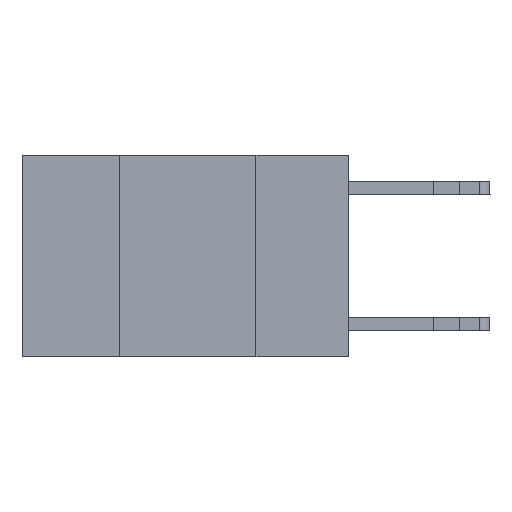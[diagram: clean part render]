
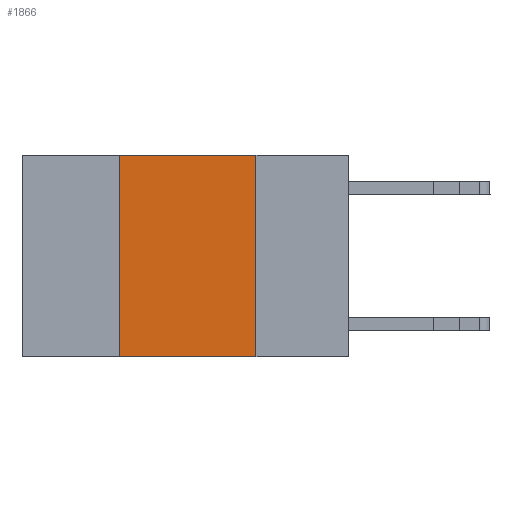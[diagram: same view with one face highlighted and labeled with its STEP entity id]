
A CAD part, left-side view. The second image highlights one B-rep face of the part: STEP entity #1866.
In plain terms, the highlighted planar face has unit normal (-1, 0, 0).
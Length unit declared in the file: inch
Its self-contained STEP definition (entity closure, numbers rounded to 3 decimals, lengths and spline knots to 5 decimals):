
#20 = CARTESIAN_POINT ( 'NONE',  ( 0., 0.42, 0. ) ) ;
#756 = ORIENTED_EDGE ( 'NONE', *, *, #8508, .F. ) ;
#1008 = LINE ( 'NONE', #17419, #14251 ) ;
#1150 = VERTEX_POINT ( 'NONE', #14821 ) ;
#1290 = LINE ( 'NONE', #5281, #10766 ) ;
#1866 = ADVANCED_FACE ( 'NONE', ( #12064 ), #17331, .F. ) ;
#2930 = EDGE_LOOP ( 'NONE', ( #5076, #9175, #756, #7237 ) ) ;
#4109 = CARTESIAN_POINT ( 'NONE',  ( 0., 0.17, 0. ) ) ;
#5074 = DIRECTION ( 'NONE',  ( 0., -1., 0. ) ) ;
#5076 = ORIENTED_EDGE ( 'NONE', *, *, #10309, .F. ) ;
#5144 = CARTESIAN_POINT ( 'NONE',  ( 0., 0.6, 0. ) ) ;
#5281 = CARTESIAN_POINT ( 'NONE',  ( 0., 0.6, -0.37 ) ) ;
#5461 = DIRECTION ( 'NONE',  ( 0., 0., -1. ) ) ;
#7237 = ORIENTED_EDGE ( 'NONE', *, *, #7477, .T. ) ;
#7477 = EDGE_CURVE ( 'NONE', #13614, #10065, #1290, .T. ) ;
#7656 = AXIS2_PLACEMENT_3D ( 'NONE', #5144, #17405, #13313 ) ;
#8288 = EDGE_CURVE ( 'NONE', #1150, #13953, #1008, .T. ) ;
#8508 = EDGE_CURVE ( 'NONE', #13614, #1150, #12174, .T. ) ;
#9175 = ORIENTED_EDGE ( 'NONE', *, *, #8288, .F. ) ;
#10065 = VERTEX_POINT ( 'NONE', #11707 ) ;
#10309 = EDGE_CURVE ( 'NONE', #13953, #10065, #12397, .T. ) ;
#10766 = VECTOR ( 'NONE', #12216, 39.37008 ) ;
#11707 = CARTESIAN_POINT ( 'NONE',  ( 0., 0.17, -0.37 ) ) ;
#12064 = FACE_OUTER_BOUND ( 'NONE', #2930, .T. ) ;
#12174 = LINE ( 'NONE', #20, #12218 ) ;
#12216 = DIRECTION ( 'NONE',  ( 0., -1., 0. ) ) ;
#12218 = VECTOR ( 'NONE', #16301, 39.37008 ) ;
#12397 = LINE ( 'NONE', #15380, #16010 ) ;
#13313 = DIRECTION ( 'NONE',  ( 0., 0., -1. ) ) ;
#13614 = VERTEX_POINT ( 'NONE', #16503 ) ;
#13953 = VERTEX_POINT ( 'NONE', #4109 ) ;
#14251 = VECTOR ( 'NONE', #5074, 39.37008 ) ;
#14821 = CARTESIAN_POINT ( 'NONE',  ( 0., 0.42, 0. ) ) ;
#15380 = CARTESIAN_POINT ( 'NONE',  ( 0., 0.17, 0. ) ) ;
#16010 = VECTOR ( 'NONE', #5461, 39.37008 ) ;
#16301 = DIRECTION ( 'NONE',  ( 0., 0., 1. ) ) ;
#16503 = CARTESIAN_POINT ( 'NONE',  ( 0., 0.42, -0.37 ) ) ;
#17331 = PLANE ( 'NONE',  #7656 ) ;
#17405 = DIRECTION ( 'NONE',  ( 1., 0., 0. ) ) ;
#17419 = CARTESIAN_POINT ( 'NONE',  ( 0., 0.6, 0. ) ) ;
